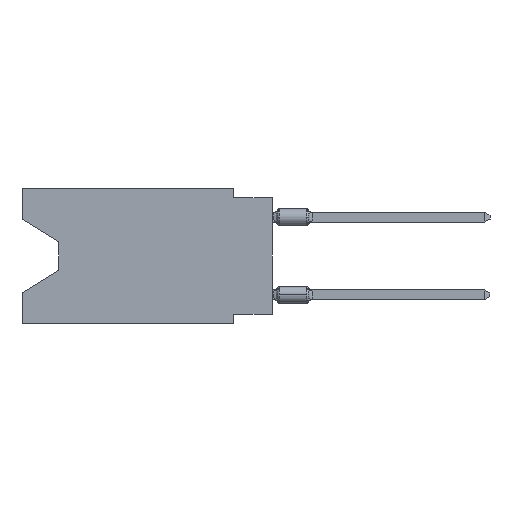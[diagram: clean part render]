
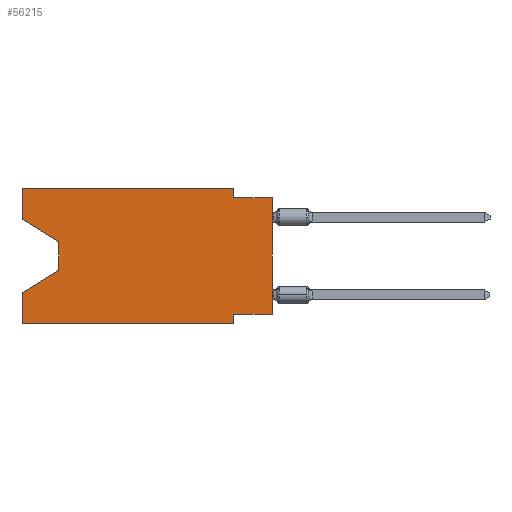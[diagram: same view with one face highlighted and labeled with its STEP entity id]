
A CAD part, left-side view. The second image highlights one B-rep face of the part: STEP entity #56215.
In plain terms, the highlighted planar face has unit normal (-1, 0, 0).
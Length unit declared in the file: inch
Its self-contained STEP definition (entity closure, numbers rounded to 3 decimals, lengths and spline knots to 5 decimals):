
#537 = CARTESIAN_POINT ( 'NONE',  ( 0., 0.1, 0. ) ) ;
#1167 = VECTOR ( 'NONE', #54964, 39.37008 ) ;
#1833 = VERTEX_POINT ( 'NONE', #49715 ) ;
#2304 = CARTESIAN_POINT ( 'NONE',  ( 0., 0., -0.025 ) ) ;
#4443 = DIRECTION ( 'NONE',  ( 0., 0., -1. ) ) ;
#5842 = FACE_OUTER_BOUND ( 'NONE', #8495, .T. ) ;
#6040 = ORIENTED_EDGE ( 'NONE', *, *, #46501, .F. ) ;
#6373 = CARTESIAN_POINT ( 'NONE',  ( 0., 0., -0.325 ) ) ;
#6870 = VERTEX_POINT ( 'NONE', #537 ) ;
#6885 = CARTESIAN_POINT ( 'NONE',  ( 0., 0.55, -0.212 ) ) ;
#7442 = VERTEX_POINT ( 'NONE', #39166 ) ;
#8495 = EDGE_LOOP ( 'NONE', ( #30726, #19165, #44553, #13390, #49327, #25196, #24434, #42468, #10069, #6040, #37749, #49908 ) ) ;
#8958 = CARTESIAN_POINT ( 'NONE',  ( 0., 0.1, 0. ) ) ;
#8996 = CARTESIAN_POINT ( 'NONE',  ( 0., 0., -0.325 ) ) ;
#10069 = ORIENTED_EDGE ( 'NONE', *, *, #57162, .F. ) ;
#10302 = DIRECTION ( 'NONE',  ( 0., 0., 1. ) ) ;
#10654 = CARTESIAN_POINT ( 'NONE',  ( 0., 0.645, 0. ) ) ;
#11472 = EDGE_CURVE ( 'NONE', #30996, #39660, #12955, .T. ) ;
#12955 = LINE ( 'NONE', #21999, #36189 ) ;
#13390 = ORIENTED_EDGE ( 'NONE', *, *, #50359, .F. ) ;
#13586 = EDGE_CURVE ( 'NONE', #47425, #20188, #40197, .T. ) ;
#14525 = LINE ( 'NONE', #33165, #34614 ) ;
#14792 = VECTOR ( 'NONE', #37000, 39.37008 ) ;
#15723 = CARTESIAN_POINT ( 'NONE',  ( 0., 0.55, -0.138 ) ) ;
#16064 = PLANE ( 'NONE',  #32895 ) ;
#17921 = DIRECTION ( 'NONE',  ( 0., 0., 1. ) ) ;
#19165 = ORIENTED_EDGE ( 'NONE', *, *, #11472, .T. ) ;
#20188 = VERTEX_POINT ( 'NONE', #50434 ) ;
#21619 = VECTOR ( 'NONE', #51268, 39.37008 ) ;
#21999 = CARTESIAN_POINT ( 'NONE',  ( 0., 0.55, -0.138 ) ) ;
#22367 = LINE ( 'NONE', #55443, #54062 ) ;
#22440 = CARTESIAN_POINT ( 'NONE',  ( 0., 0.645, 0. ) ) ;
#22927 = EDGE_CURVE ( 'NONE', #38313, #7442, #56053, .T. ) ;
#24434 = ORIENTED_EDGE ( 'NONE', *, *, #44076, .F. ) ;
#25196 = ORIENTED_EDGE ( 'NONE', *, *, #56770, .F. ) ;
#25235 = VERTEX_POINT ( 'NONE', #8996 ) ;
#25614 = VECTOR ( 'NONE', #4443, 39.37008 ) ;
#28356 = VECTOR ( 'NONE', #49471, 39.37008 ) ;
#28406 = CARTESIAN_POINT ( 'NONE',  ( 0., 0.645, -0.26975 ) ) ;
#28605 = LINE ( 'NONE', #55970, #36797 ) ;
#29158 = LINE ( 'NONE', #6885, #54041 ) ;
#29649 = VERTEX_POINT ( 'NONE', #51752 ) ;
#30726 = ORIENTED_EDGE ( 'NONE', *, *, #56285, .T. ) ;
#30996 = VERTEX_POINT ( 'NONE', #15723 ) ;
#31300 = DIRECTION ( 'NONE',  ( 0., 0., -1. ) ) ;
#31702 = CARTESIAN_POINT ( 'NONE',  ( 0., 0.55, -0.212 ) ) ;
#31836 = LINE ( 'NONE', #8958, #25614 ) ;
#32895 = AXIS2_PLACEMENT_3D ( 'NONE', #10654, #34414, #52441 ) ;
#33165 = CARTESIAN_POINT ( 'NONE',  ( 0., 0.645, 0. ) ) ;
#34082 = CARTESIAN_POINT ( 'NONE',  ( 0., 0.645, -0.35 ) ) ;
#34414 = DIRECTION ( 'NONE',  ( 1., 0., 0. ) ) ;
#34614 = VECTOR ( 'NONE', #10302, 39.37008 ) ;
#34782 = LINE ( 'NONE', #39587, #28356 ) ;
#35435 = VECTOR ( 'NONE', #17921, 39.37008 ) ;
#36189 = VECTOR ( 'NONE', #31300, 39.37008 ) ;
#36797 = VECTOR ( 'NONE', #37327, 39.37008 ) ;
#36904 = CARTESIAN_POINT ( 'NONE',  ( 0., 0.645, -0.08025 ) ) ;
#37000 = DIRECTION ( 'NONE',  ( 0., 0., 1. ) ) ;
#37327 = DIRECTION ( 'NONE',  ( 0., -1., 0. ) ) ;
#37602 = CARTESIAN_POINT ( 'NONE',  ( 0., 0., 0. ) ) ;
#37749 = ORIENTED_EDGE ( 'NONE', *, *, #44647, .F. ) ;
#38313 = VERTEX_POINT ( 'NONE', #59352 ) ;
#39166 = CARTESIAN_POINT ( 'NONE',  ( 0., 0.1, -0.35 ) ) ;
#39587 = CARTESIAN_POINT ( 'NONE',  ( 0., 0.645, 0. ) ) ;
#39660 = VERTEX_POINT ( 'NONE', #31702 ) ;
#39869 = VECTOR ( 'NONE', #51529, 39.37008 ) ;
#40197 = LINE ( 'NONE', #22440, #35435 ) ;
#41125 = LINE ( 'NONE', #36904, #1167 ) ;
#42468 = ORIENTED_EDGE ( 'NONE', *, *, #43270, .T. ) ;
#43078 = LINE ( 'NONE', #6373, #21619 ) ;
#43270 = EDGE_CURVE ( 'NONE', #25235, #45720, #55954, .T. ) ;
#44076 = EDGE_CURVE ( 'NONE', #25235, #1833, #43078, .T. ) ;
#44553 = ORIENTED_EDGE ( 'NONE', *, *, #54145, .T. ) ;
#44647 = EDGE_CURVE ( 'NONE', #20188, #6870, #34782, .T. ) ;
#45220 = DIRECTION ( 'NONE',  ( 0., 0., -1. ) ) ;
#45720 = VERTEX_POINT ( 'NONE', #2304 ) ;
#46501 = EDGE_CURVE ( 'NONE', #6870, #29649, #31836, .T. ) ;
#47425 = VERTEX_POINT ( 'NONE', #49421 ) ;
#48611 = VERTEX_POINT ( 'NONE', #28406 ) ;
#49327 = ORIENTED_EDGE ( 'NONE', *, *, #22927, .T. ) ;
#49421 = CARTESIAN_POINT ( 'NONE',  ( 0., 0.645, -0.08025 ) ) ;
#49471 = DIRECTION ( 'NONE',  ( 0., -1., 0. ) ) ;
#49715 = CARTESIAN_POINT ( 'NONE',  ( 0., 0.1, -0.325 ) ) ;
#49908 = ORIENTED_EDGE ( 'NONE', *, *, #13586, .F. ) ;
#50359 = EDGE_CURVE ( 'NONE', #38313, #48611, #14525, .T. ) ;
#50434 = CARTESIAN_POINT ( 'NONE',  ( 0., 0.645, 0. ) ) ;
#51268 = DIRECTION ( 'NONE',  ( 0., 1., 0. ) ) ;
#51529 = DIRECTION ( 'NONE',  ( 0., -1., 0. ) ) ;
#51752 = CARTESIAN_POINT ( 'NONE',  ( 0., 0.1, -0.025 ) ) ;
#52441 = DIRECTION ( 'NONE',  ( 0., 0., -1. ) ) ;
#52618 = DIRECTION ( 'NONE',  ( 0., 0.855, -0.519 ) ) ;
#54041 = VECTOR ( 'NONE', #52618, 39.37008 ) ;
#54062 = VECTOR ( 'NONE', #45220, 39.37008 ) ;
#54145 = EDGE_CURVE ( 'NONE', #39660, #48611, #29158, .T. ) ;
#54964 = DIRECTION ( 'NONE',  ( 0., -0.855, -0.519 ) ) ;
#55443 = CARTESIAN_POINT ( 'NONE',  ( 0., 0.1, -0.35 ) ) ;
#55954 = LINE ( 'NONE', #37602, #14792 ) ;
#55970 = CARTESIAN_POINT ( 'NONE',  ( 0., 0., -0.025 ) ) ;
#56053 = LINE ( 'NONE', #34082, #39869 ) ;
#56215 = ADVANCED_FACE ( 'NONE', ( #5842 ), #16064, .F. ) ;
#56285 = EDGE_CURVE ( 'NONE', #47425, #30996, #41125, .T. ) ;
#56770 = EDGE_CURVE ( 'NONE', #1833, #7442, #22367, .T. ) ;
#57162 = EDGE_CURVE ( 'NONE', #29649, #45720, #28605, .T. ) ;
#59352 = CARTESIAN_POINT ( 'NONE',  ( 0., 0.645, -0.35 ) ) ;
